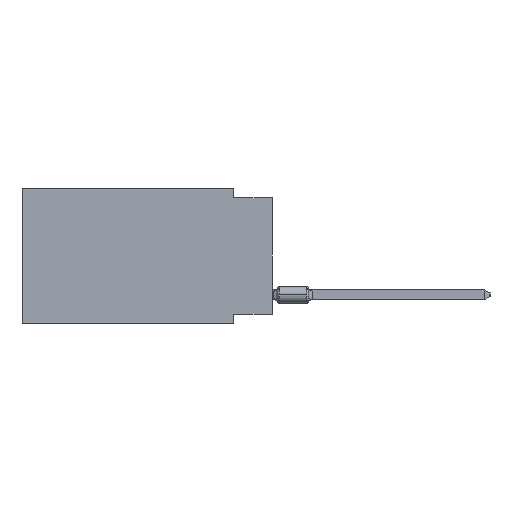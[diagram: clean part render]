
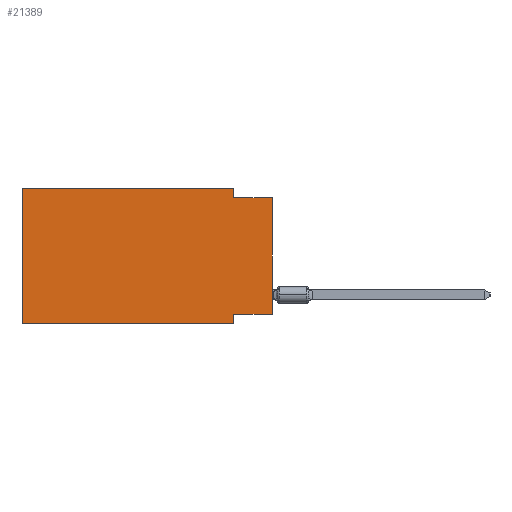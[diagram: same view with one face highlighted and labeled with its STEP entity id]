
A CAD part, left-side view. The second image highlights one B-rep face of the part: STEP entity #21389.
In plain terms, the highlighted planar face has unit normal (-1, 0, 0).
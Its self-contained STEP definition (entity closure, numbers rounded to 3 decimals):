
#11 = CARTESIAN_POINT ( 'NONE',  ( 0., 16.383, 0. ) ) ;
#969 = EDGE_CURVE ( 'NONE', #13008, #14328, #27104, .T. ) ;
#2271 = LINE ( 'NONE', #13326, #5249 ) ;
#3345 = ORIENTED_EDGE ( 'NONE', *, *, #969, .T. ) ;
#4851 = ORIENTED_EDGE ( 'NONE', *, *, #59099, .F. ) ;
#5249 = VECTOR ( 'NONE', #43415, 1000. ) ;
#5792 = LINE ( 'NONE', #36559, #11721 ) ;
#5835 = CARTESIAN_POINT ( 'NONE',  ( 0., 0., -8.255 ) ) ;
#6373 = LINE ( 'NONE', #26790, #15373 ) ;
#7516 = CARTESIAN_POINT ( 'NONE',  ( 0., 0., -8.255 ) ) ;
#8913 = CARTESIAN_POINT ( 'NONE',  ( 0., 2.54, -8.89 ) ) ;
#11721 = VECTOR ( 'NONE', #57883, 1000. ) ;
#12715 = DIRECTION ( 'NONE',  ( 0., -1., 0. ) ) ;
#12887 = VERTEX_POINT ( 'NONE', #30873 ) ;
#13008 = VERTEX_POINT ( 'NONE', #17799 ) ;
#13311 = DIRECTION ( 'NONE',  ( 1., 0., 0. ) ) ;
#13326 = CARTESIAN_POINT ( 'NONE',  ( 0., 16.383, 0. ) ) ;
#14328 = VERTEX_POINT ( 'NONE', #8913 ) ;
#15373 = VECTOR ( 'NONE', #15771, 1000. ) ;
#15575 = VERTEX_POINT ( 'NONE', #25209 ) ;
#15771 = DIRECTION ( 'NONE',  ( 0., 0., 1. ) ) ;
#17799 = CARTESIAN_POINT ( 'NONE',  ( 0., 16.383, -8.89 ) ) ;
#18061 = VECTOR ( 'NONE', #12715, 1000. ) ;
#18072 = CARTESIAN_POINT ( 'NONE',  ( 0., 16.383, -8.89 ) ) ;
#21389 = ADVANCED_FACE ( 'NONE', ( #33026 ), #43728, .F. ) ;
#22133 = CARTESIAN_POINT ( 'NONE',  ( 0., 16.383, 0. ) ) ;
#22776 = CARTESIAN_POINT ( 'NONE',  ( 0., 0., -0.635 ) ) ;
#22792 = LINE ( 'NONE', #22133, #54445 ) ;
#22980 = ORIENTED_EDGE ( 'NONE', *, *, #44910, .F. ) ;
#23561 = ORIENTED_EDGE ( 'NONE', *, *, #63049, .F. ) ;
#23802 = VECTOR ( 'NONE', #59302, 1000. ) ;
#25209 = CARTESIAN_POINT ( 'NONE',  ( 0., 2.54, -0.635 ) ) ;
#25965 = EDGE_CURVE ( 'NONE', #30010, #12887, #22792, .T. ) ;
#26790 = CARTESIAN_POINT ( 'NONE',  ( 0., 0., 0. ) ) ;
#27104 = LINE ( 'NONE', #18072, #18061 ) ;
#29080 = ORIENTED_EDGE ( 'NONE', *, *, #25965, .F. ) ;
#30010 = VERTEX_POINT ( 'NONE', #11 ) ;
#30668 = AXIS2_PLACEMENT_3D ( 'NONE', #38712, #13311, #33698 ) ;
#30873 = CARTESIAN_POINT ( 'NONE',  ( 0., 2.54, 0. ) ) ;
#32830 = VERTEX_POINT ( 'NONE', #42032 ) ;
#33026 = FACE_OUTER_BOUND ( 'NONE', #34450, .T. ) ;
#33698 = DIRECTION ( 'NONE',  ( 0., 0., -1. ) ) ;
#34450 = EDGE_LOOP ( 'NONE', ( #63983, #23561, #22980, #29080, #58258, #3345, #4851, #42351 ) ) ;
#36491 = VECTOR ( 'NONE', #63488, 1000. ) ;
#36559 = CARTESIAN_POINT ( 'NONE',  ( 0., 2.54, 0. ) ) ;
#37919 = EDGE_CURVE ( 'NONE', #61544, #32830, #64625, .T. ) ;
#38608 = EDGE_CURVE ( 'NONE', #61544, #57861, #6373, .T. ) ;
#38712 = CARTESIAN_POINT ( 'NONE',  ( 0., 16.383, 0. ) ) ;
#41841 = CARTESIAN_POINT ( 'NONE',  ( 0., 2.54, -8.89 ) ) ;
#42032 = CARTESIAN_POINT ( 'NONE',  ( 0., 2.54, -8.255 ) ) ;
#42351 = ORIENTED_EDGE ( 'NONE', *, *, #37919, .F. ) ;
#42493 = LINE ( 'NONE', #22776, #36491 ) ;
#43170 = DIRECTION ( 'NONE',  ( 0., -1., 0. ) ) ;
#43415 = DIRECTION ( 'NONE',  ( 0., 0., 1. ) ) ;
#43630 = CARTESIAN_POINT ( 'NONE',  ( 0., 0., -0.635 ) ) ;
#43728 = PLANE ( 'NONE',  #30668 ) ;
#44910 = EDGE_CURVE ( 'NONE', #12887, #15575, #5792, .T. ) ;
#47852 = VECTOR ( 'NONE', #51553, 1000. ) ;
#51553 = DIRECTION ( 'NONE',  ( 0., 0., -1. ) ) ;
#54445 = VECTOR ( 'NONE', #43170, 1000. ) ;
#57501 = LINE ( 'NONE', #41841, #47852 ) ;
#57861 = VERTEX_POINT ( 'NONE', #43630 ) ;
#57883 = DIRECTION ( 'NONE',  ( 0., 0., -1. ) ) ;
#58258 = ORIENTED_EDGE ( 'NONE', *, *, #59653, .F. ) ;
#59099 = EDGE_CURVE ( 'NONE', #32830, #14328, #57501, .T. ) ;
#59302 = DIRECTION ( 'NONE',  ( 0., 1., 0. ) ) ;
#59653 = EDGE_CURVE ( 'NONE', #13008, #30010, #2271, .T. ) ;
#61544 = VERTEX_POINT ( 'NONE', #5835 ) ;
#63049 = EDGE_CURVE ( 'NONE', #15575, #57861, #42493, .T. ) ;
#63488 = DIRECTION ( 'NONE',  ( 0., -1., 0. ) ) ;
#63983 = ORIENTED_EDGE ( 'NONE', *, *, #38608, .T. ) ;
#64625 = LINE ( 'NONE', #7516, #23802 ) ;
